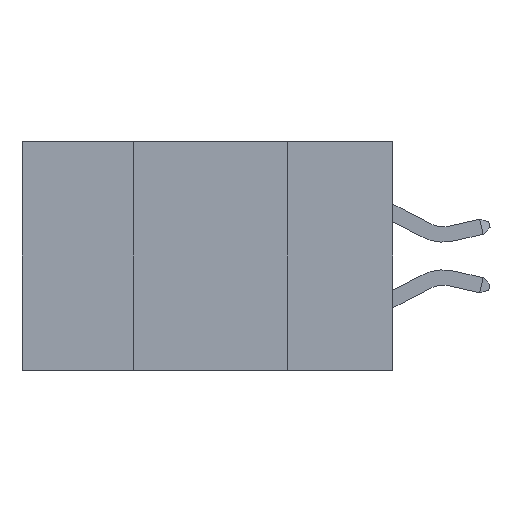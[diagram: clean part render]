
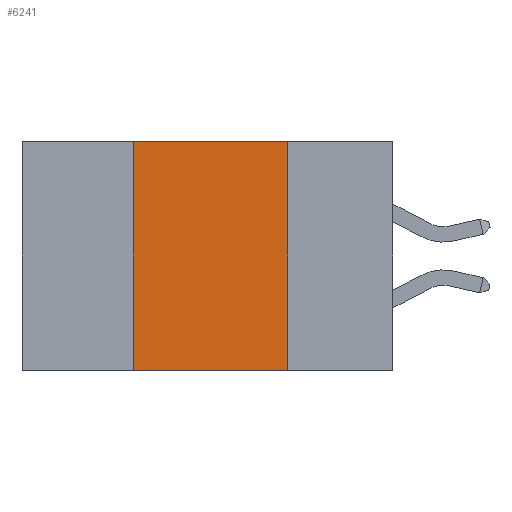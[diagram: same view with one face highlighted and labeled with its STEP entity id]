
A CAD part, left-side view. The second image highlights one B-rep face of the part: STEP entity #6241.
In plain terms, the highlighted planar face has unit normal (-1, 0, 0).
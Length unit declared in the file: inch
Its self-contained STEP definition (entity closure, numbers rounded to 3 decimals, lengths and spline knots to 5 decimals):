
#681 = DIRECTION ( 'NONE',  ( 0., -1., 0. ) ) ;
#784 = DIRECTION ( 'NONE',  ( 0., 0., -1. ) ) ;
#815 = LINE ( 'NONE', #3535, #8202 ) ;
#1084 = CARTESIAN_POINT ( 'NONE',  ( 0., 0.42, 0. ) ) ;
#1114 = DIRECTION ( 'NONE',  ( 1., 0., 0. ) ) ;
#1173 = VECTOR ( 'NONE', #9755, 39.37008 ) ;
#2215 = VERTEX_POINT ( 'NONE', #8178 ) ;
#2279 = LINE ( 'NONE', #10184, #9605 ) ;
#2829 = EDGE_CURVE ( 'NONE', #7031, #5640, #3746, .T. ) ;
#3090 = CARTESIAN_POINT ( 'NONE',  ( 0., 0.42, 0. ) ) ;
#3361 = EDGE_LOOP ( 'NONE', ( #8239, #3452, #5616, #11451 ) ) ;
#3452 = ORIENTED_EDGE ( 'NONE', *, *, #5259, .F. ) ;
#3535 = CARTESIAN_POINT ( 'NONE',  ( 0., 0.6, 0. ) ) ;
#3746 = LINE ( 'NONE', #3090, #1173 ) ;
#4820 = CARTESIAN_POINT ( 'NONE',  ( 0., 0.6, 0. ) ) ;
#5259 = EDGE_CURVE ( 'NONE', #5640, #2215, #815, .T. ) ;
#5616 = ORIENTED_EDGE ( 'NONE', *, *, #2829, .F. ) ;
#5640 = VERTEX_POINT ( 'NONE', #1084 ) ;
#6241 = ADVANCED_FACE ( 'NONE', ( #8901 ), #11547, .F. ) ;
#6336 = DIRECTION ( 'NONE',  ( 0., -1., 0. ) ) ;
#6537 = CARTESIAN_POINT ( 'NONE',  ( 0., 0.17, 0. ) ) ;
#7031 = VERTEX_POINT ( 'NONE', #10224 ) ;
#7763 = DIRECTION ( 'NONE',  ( 0., 0., -1. ) ) ;
#8066 = EDGE_CURVE ( 'NONE', #2215, #11707, #12011, .T. ) ;
#8178 = CARTESIAN_POINT ( 'NONE',  ( 0., 0.17, 0. ) ) ;
#8202 = VECTOR ( 'NONE', #6336, 39.37008 ) ;
#8239 = ORIENTED_EDGE ( 'NONE', *, *, #8066, .F. ) ;
#8729 = VECTOR ( 'NONE', #784, 39.37008 ) ;
#8901 = FACE_OUTER_BOUND ( 'NONE', #3361, .T. ) ;
#9413 = CARTESIAN_POINT ( 'NONE',  ( 0., 0.17, -0.37 ) ) ;
#9605 = VECTOR ( 'NONE', #681, 39.37008 ) ;
#9755 = DIRECTION ( 'NONE',  ( 0., 0., 1. ) ) ;
#10184 = CARTESIAN_POINT ( 'NONE',  ( 0., 0.6, -0.37 ) ) ;
#10224 = CARTESIAN_POINT ( 'NONE',  ( 0., 0.42, -0.37 ) ) ;
#11451 = ORIENTED_EDGE ( 'NONE', *, *, #12182, .T. ) ;
#11547 = PLANE ( 'NONE',  #11806 ) ;
#11707 = VERTEX_POINT ( 'NONE', #9413 ) ;
#11806 = AXIS2_PLACEMENT_3D ( 'NONE', #4820, #1114, #7763 ) ;
#12011 = LINE ( 'NONE', #6537, #8729 ) ;
#12182 = EDGE_CURVE ( 'NONE', #7031, #11707, #2279, .T. ) ;
